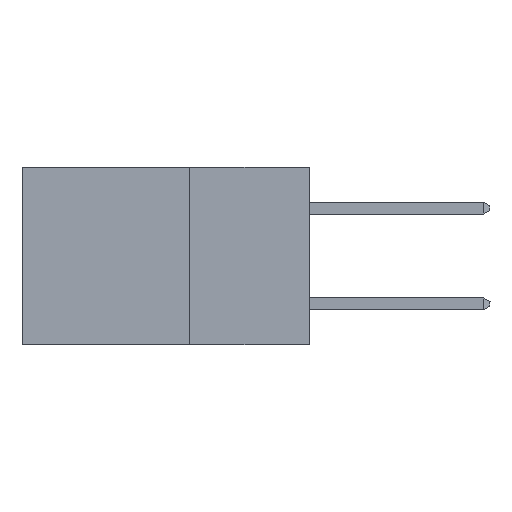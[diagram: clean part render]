
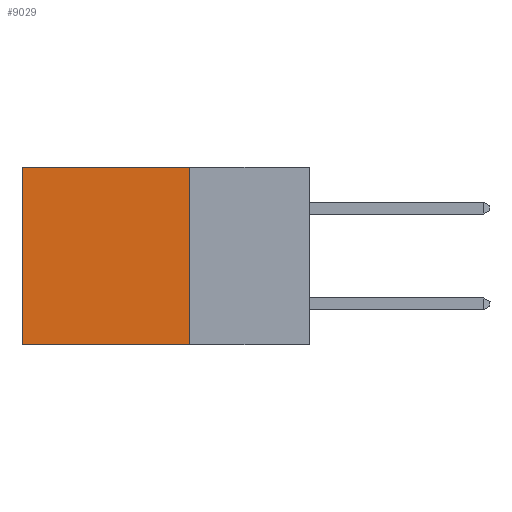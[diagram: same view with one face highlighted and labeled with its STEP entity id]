
A CAD part, left-side view. The second image highlights one B-rep face of the part: STEP entity #9029.
In plain terms, the highlighted planar face has unit normal (-1, 0, 0).
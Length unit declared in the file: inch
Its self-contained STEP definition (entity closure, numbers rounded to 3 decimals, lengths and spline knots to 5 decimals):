
#458 = LINE ( 'NONE', #37395, #10567 ) ;
#2043 = EDGE_CURVE ( 'NONE', #42119, #35339, #32366, .T. ) ;
#3964 = DIRECTION ( 'NONE',  ( 0., 0., -1. ) ) ;
#9029 = ADVANCED_FACE ( 'NONE', ( #33281 ), #12756, .F. ) ;
#9976 = CARTESIAN_POINT ( 'NONE',  ( 0.2875, 0.25, -0.37 ) ) ;
#10567 = VECTOR ( 'NONE', #3964, 39.37008 ) ;
#12756 = PLANE ( 'NONE',  #34979 ) ;
#14033 = ORIENTED_EDGE ( 'NONE', *, *, #26219, .T. ) ;
#14565 = EDGE_CURVE ( 'NONE', #42119, #35184, #18393, .T. ) ;
#18393 = LINE ( 'NONE', #28027, #31647 ) ;
#18464 = CARTESIAN_POINT ( 'NONE',  ( 0.2875, 0.6, -0.37 ) ) ;
#19940 = EDGE_CURVE ( 'NONE', #35339, #33782, #32894, .T. ) ;
#20441 = ORIENTED_EDGE ( 'NONE', *, *, #19940, .F. ) ;
#21754 = EDGE_LOOP ( 'NONE', ( #14033, #20441, #25732, #40543 ) ) ;
#23015 = DIRECTION ( 'NONE',  ( 0., 0., -1. ) ) ;
#25732 = ORIENTED_EDGE ( 'NONE', *, *, #2043, .F. ) ;
#25890 = DIRECTION ( 'NONE',  ( 1., 0., 0. ) ) ;
#26219 = EDGE_CURVE ( 'NONE', #35184, #33782, #458, .T. ) ;
#26973 = CARTESIAN_POINT ( 'NONE',  ( 0.2875, 0.25, -0.37 ) ) ;
#28027 = CARTESIAN_POINT ( 'NONE',  ( 0.2875, 0.25, 0. ) ) ;
#29089 = CARTESIAN_POINT ( 'NONE',  ( 0.2875, 0.25, 0. ) ) ;
#31527 = CARTESIAN_POINT ( 'NONE',  ( 0.2875, 0.25, 0. ) ) ;
#31647 = VECTOR ( 'NONE', #38284, 39.37008 ) ;
#32366 = LINE ( 'NONE', #29089, #40644 ) ;
#32894 = LINE ( 'NONE', #26973, #34725 ) ;
#33281 = FACE_OUTER_BOUND ( 'NONE', #21754, .T. ) ;
#33782 = VERTEX_POINT ( 'NONE', #18464 ) ;
#34725 = VECTOR ( 'NONE', #36813, 39.37008 ) ;
#34979 = AXIS2_PLACEMENT_3D ( 'NONE', #40059, #25890, #23015 ) ;
#35184 = VERTEX_POINT ( 'NONE', #38853 ) ;
#35339 = VERTEX_POINT ( 'NONE', #9976 ) ;
#35864 = DIRECTION ( 'NONE',  ( 0., 0., -1. ) ) ;
#36813 = DIRECTION ( 'NONE',  ( 0., 1., 0. ) ) ;
#37395 = CARTESIAN_POINT ( 'NONE',  ( 0.2875, 0.6, 0. ) ) ;
#38284 = DIRECTION ( 'NONE',  ( 0., 1., 0. ) ) ;
#38853 = CARTESIAN_POINT ( 'NONE',  ( 0.2875, 0.6, 0. ) ) ;
#40059 = CARTESIAN_POINT ( 'NONE',  ( 0.2875, 0.25, 0. ) ) ;
#40543 = ORIENTED_EDGE ( 'NONE', *, *, #14565, .T. ) ;
#40644 = VECTOR ( 'NONE', #35864, 39.37008 ) ;
#42119 = VERTEX_POINT ( 'NONE', #31527 ) ;
